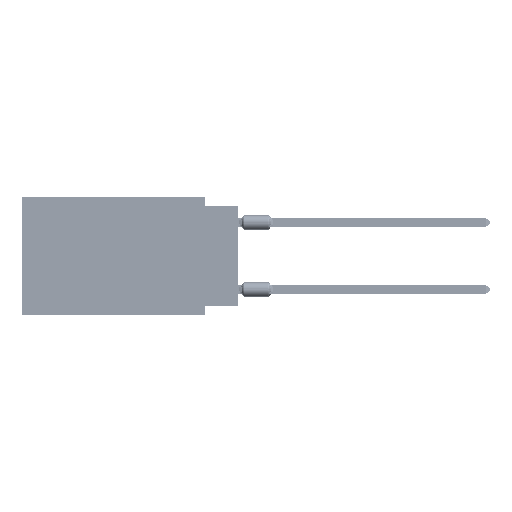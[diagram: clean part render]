
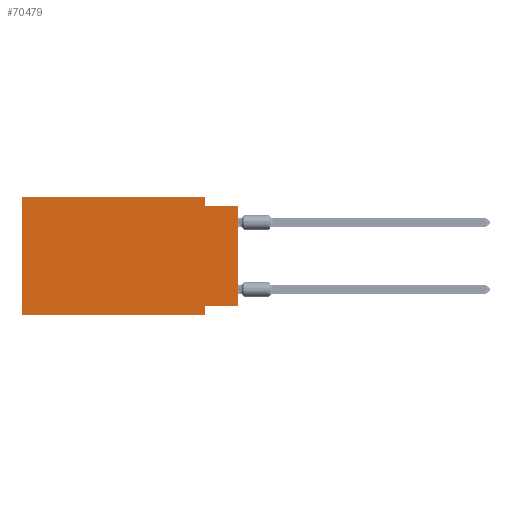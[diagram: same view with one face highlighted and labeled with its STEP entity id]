
A CAD part, left-side view. The second image highlights one B-rep face of the part: STEP entity #70479.
In plain terms, the highlighted planar face has unit normal (-1, 0, 0).
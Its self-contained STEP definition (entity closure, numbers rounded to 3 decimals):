
#153 = DIRECTION ( 'NONE',  ( 0., 0., -1. ) ) ;
#712 = EDGE_CURVE ( 'NONE', #67496, #92335, #86823, .T. ) ;
#5820 = EDGE_CURVE ( 'NONE', #8862, #22287, #36791, .T. ) ;
#6996 = DIRECTION ( 'NONE',  ( 0., 0., 1. ) ) ;
#8218 = CARTESIAN_POINT ( 'NONE',  ( 0., 2.54, -8.89 ) ) ;
#8794 = DIRECTION ( 'NONE',  ( 0., 0., -1. ) ) ;
#8862 = VERTEX_POINT ( 'NONE', #77036 ) ;
#10377 = EDGE_CURVE ( 'NONE', #8862, #67496, #11345, .T. ) ;
#11324 = VECTOR ( 'NONE', #6996, 1000. ) ;
#11345 = LINE ( 'NONE', #84378, #69781 ) ;
#13665 = VECTOR ( 'NONE', #8794, 1000. ) ;
#14310 = LINE ( 'NONE', #46632, #11324 ) ;
#14518 = VECTOR ( 'NONE', #52876, 1000. ) ;
#17809 = VERTEX_POINT ( 'NONE', #56789 ) ;
#18157 = EDGE_CURVE ( 'NONE', #17809, #57747, #14310, .T. ) ;
#20804 = DIRECTION ( 'NONE',  ( 1., 0., 0. ) ) ;
#21677 = ORIENTED_EDGE ( 'NONE', *, *, #18157, .F. ) ;
#22287 = VERTEX_POINT ( 'NONE', #92067 ) ;
#22704 = EDGE_LOOP ( 'NONE', ( #33076, #59133, #76493, #75473, #21677, #79109, #61074, #27069 ) ) ;
#27069 = ORIENTED_EDGE ( 'NONE', *, *, #10377, .F. ) ;
#27186 = VERTEX_POINT ( 'NONE', #94798 ) ;
#32242 = LINE ( 'NONE', #63612, #13665 ) ;
#32579 = VECTOR ( 'NONE', #84302, 1000. ) ;
#33076 = ORIENTED_EDGE ( 'NONE', *, *, #5820, .T. ) ;
#36435 = DIRECTION ( 'NONE',  ( 0., 0., -1. ) ) ;
#36755 = EDGE_CURVE ( 'NONE', #27186, #92765, #32242, .T. ) ;
#36791 = LINE ( 'NONE', #44612, #32579 ) ;
#39168 = CARTESIAN_POINT ( 'NONE',  ( 0., 16.383, 0. ) ) ;
#44175 = DIRECTION ( 'NONE',  ( 0., 1., 0. ) ) ;
#44612 = CARTESIAN_POINT ( 'NONE',  ( 0., 0., 0. ) ) ;
#44940 = EDGE_CURVE ( 'NONE', #92765, #22287, #62819, .T. ) ;
#46632 = CARTESIAN_POINT ( 'NONE',  ( 0., 16.383, 0. ) ) ;
#50315 = VECTOR ( 'NONE', #89483, 1000. ) ;
#51089 = FACE_OUTER_BOUND ( 'NONE', #22704, .T. ) ;
#52021 = EDGE_CURVE ( 'NONE', #17809, #92335, #54428, .T. ) ;
#52113 = CARTESIAN_POINT ( 'NONE',  ( 0., 16.383, 0. ) ) ;
#52876 = DIRECTION ( 'NONE',  ( 0., -1., 0. ) ) ;
#54428 = LINE ( 'NONE', #71129, #14518 ) ;
#55184 = VECTOR ( 'NONE', #71691, 1000. ) ;
#55523 = CARTESIAN_POINT ( 'NONE',  ( 0., 0., -0.635 ) ) ;
#56789 = CARTESIAN_POINT ( 'NONE',  ( 0., 16.383, -8.89 ) ) ;
#57140 = CARTESIAN_POINT ( 'NONE',  ( 0., 16.383, 0. ) ) ;
#57747 = VERTEX_POINT ( 'NONE', #39168 ) ;
#59133 = ORIENTED_EDGE ( 'NONE', *, *, #44940, .F. ) ;
#61074 = ORIENTED_EDGE ( 'NONE', *, *, #712, .F. ) ;
#62279 = CARTESIAN_POINT ( 'NONE',  ( 0., 2.54, -8.89 ) ) ;
#62819 = LINE ( 'NONE', #55523, #55184 ) ;
#63207 = AXIS2_PLACEMENT_3D ( 'NONE', #52113, #20804, #36435 ) ;
#63612 = CARTESIAN_POINT ( 'NONE',  ( 0., 2.54, 0. ) ) ;
#67496 = VERTEX_POINT ( 'NONE', #77466 ) ;
#69781 = VECTOR ( 'NONE', #44175, 1000. ) ;
#70479 = ADVANCED_FACE ( 'NONE', ( #51089 ), #92300, .F. ) ;
#71129 = CARTESIAN_POINT ( 'NONE',  ( 0., 16.383, -8.89 ) ) ;
#71691 = DIRECTION ( 'NONE',  ( 0., -1., 0. ) ) ;
#75473 = ORIENTED_EDGE ( 'NONE', *, *, #86392, .F. ) ;
#76493 = ORIENTED_EDGE ( 'NONE', *, *, #36755, .F. ) ;
#76934 = VECTOR ( 'NONE', #153, 1000. ) ;
#77036 = CARTESIAN_POINT ( 'NONE',  ( 0., 0., -8.255 ) ) ;
#77466 = CARTESIAN_POINT ( 'NONE',  ( 0., 2.54, -8.255 ) ) ;
#79109 = ORIENTED_EDGE ( 'NONE', *, *, #52021, .T. ) ;
#84302 = DIRECTION ( 'NONE',  ( 0., 0., 1. ) ) ;
#84378 = CARTESIAN_POINT ( 'NONE',  ( 0., 0., -8.255 ) ) ;
#86392 = EDGE_CURVE ( 'NONE', #57747, #27186, #96822, .T. ) ;
#86823 = LINE ( 'NONE', #62279, #76934 ) ;
#89483 = DIRECTION ( 'NONE',  ( 0., -1., 0. ) ) ;
#92067 = CARTESIAN_POINT ( 'NONE',  ( 0., 0., -0.635 ) ) ;
#92300 = PLANE ( 'NONE',  #63207 ) ;
#92335 = VERTEX_POINT ( 'NONE', #8218 ) ;
#92765 = VERTEX_POINT ( 'NONE', #96674 ) ;
#94798 = CARTESIAN_POINT ( 'NONE',  ( 0., 2.54, 0. ) ) ;
#96674 = CARTESIAN_POINT ( 'NONE',  ( 0., 2.54, -0.635 ) ) ;
#96822 = LINE ( 'NONE', #57140, #50315 ) ;
